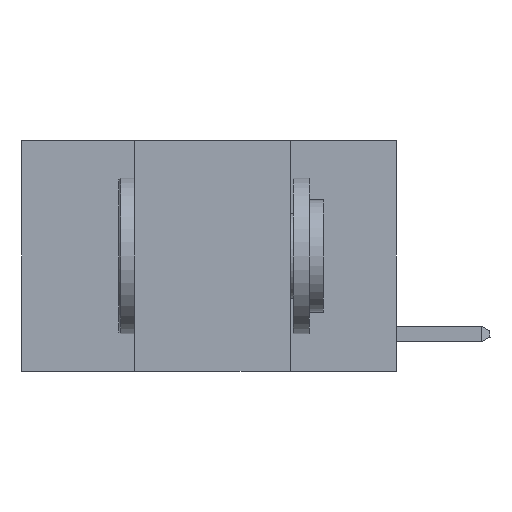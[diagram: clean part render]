
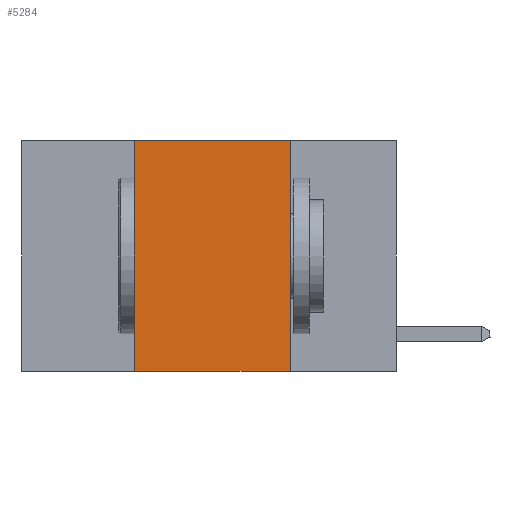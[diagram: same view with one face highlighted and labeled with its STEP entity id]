
A CAD part, left-side view. The second image highlights one B-rep face of the part: STEP entity #5284.
In plain terms, the highlighted planar face has unit normal (-1, 0, 0).
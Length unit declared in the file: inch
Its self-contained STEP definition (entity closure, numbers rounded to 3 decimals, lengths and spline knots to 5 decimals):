
#418 = CARTESIAN_POINT ( 'NONE',  ( 0., 0.6, 0. ) ) ;
#1654 = EDGE_CURVE ( 'NONE', #6541, #2169, #10097, .T. ) ;
#2167 = LINE ( 'NONE', #2624, #6141 ) ;
#2169 = VERTEX_POINT ( 'NONE', #9355 ) ;
#2624 = CARTESIAN_POINT ( 'NONE',  ( 0., 0.6, 0. ) ) ;
#2635 = CARTESIAN_POINT ( 'NONE',  ( 0., 0.17, 0. ) ) ;
#2928 = DIRECTION ( 'NONE',  ( 0., 0., -1. ) ) ;
#3011 = VECTOR ( 'NONE', #3073, 39.37008 ) ;
#3073 = DIRECTION ( 'NONE',  ( 0., -1., 0. ) ) ;
#3089 = VERTEX_POINT ( 'NONE', #2635 ) ;
#3503 = EDGE_LOOP ( 'NONE', ( #7737, #7758, #7777, #7809 ) ) ;
#3850 = VECTOR ( 'NONE', #4837, 39.37008 ) ;
#3887 = LINE ( 'NONE', #9469, #7874 ) ;
#3973 = DIRECTION ( 'NONE',  ( 0., 0., -1. ) ) ;
#4837 = DIRECTION ( 'NONE',  ( 0., 0., 1. ) ) ;
#4999 = EDGE_CURVE ( 'NONE', #2169, #3089, #2167, .T. ) ;
#5106 = CARTESIAN_POINT ( 'NONE',  ( 0., 0.17, -0.37 ) ) ;
#5122 = LINE ( 'NONE', #6221, #3011 ) ;
#5284 = ADVANCED_FACE ( 'NONE', ( #8117 ), #6885, .F. ) ;
#5793 = VERTEX_POINT ( 'NONE', #5106 ) ;
#6141 = VECTOR ( 'NONE', #7373, 39.37008 ) ;
#6221 = CARTESIAN_POINT ( 'NONE',  ( 0., 0.6, -0.37 ) ) ;
#6541 = VERTEX_POINT ( 'NONE', #8456 ) ;
#6885 = PLANE ( 'NONE',  #8569 ) ;
#7291 = EDGE_CURVE ( 'NONE', #6541, #5793, #5122, .T. ) ;
#7373 = DIRECTION ( 'NONE',  ( 0., -1., 0. ) ) ;
#7693 = DIRECTION ( 'NONE',  ( 1., 0., 0. ) ) ;
#7737 = ORIENTED_EDGE ( 'NONE', *, *, #8958, .F. ) ;
#7758 = ORIENTED_EDGE ( 'NONE', *, *, #4999, .F. ) ;
#7777 = ORIENTED_EDGE ( 'NONE', *, *, #1654, .F. ) ;
#7809 = ORIENTED_EDGE ( 'NONE', *, *, #7291, .T. ) ;
#7874 = VECTOR ( 'NONE', #3973, 39.37008 ) ;
#7989 = CARTESIAN_POINT ( 'NONE',  ( 0., 0.42, 0. ) ) ;
#8117 = FACE_OUTER_BOUND ( 'NONE', #3503, .T. ) ;
#8456 = CARTESIAN_POINT ( 'NONE',  ( 0., 0.42, -0.37 ) ) ;
#8569 = AXIS2_PLACEMENT_3D ( 'NONE', #418, #7693, #2928 ) ;
#8958 = EDGE_CURVE ( 'NONE', #3089, #5793, #3887, .T. ) ;
#9355 = CARTESIAN_POINT ( 'NONE',  ( 0., 0.42, 0. ) ) ;
#9469 = CARTESIAN_POINT ( 'NONE',  ( 0., 0.17, 0. ) ) ;
#10097 = LINE ( 'NONE', #7989, #3850 ) ;
